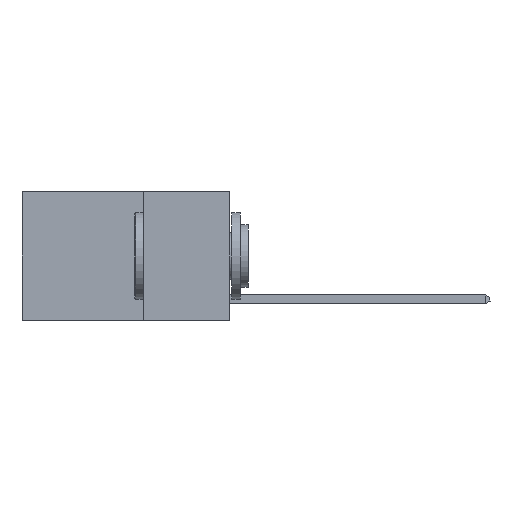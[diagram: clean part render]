
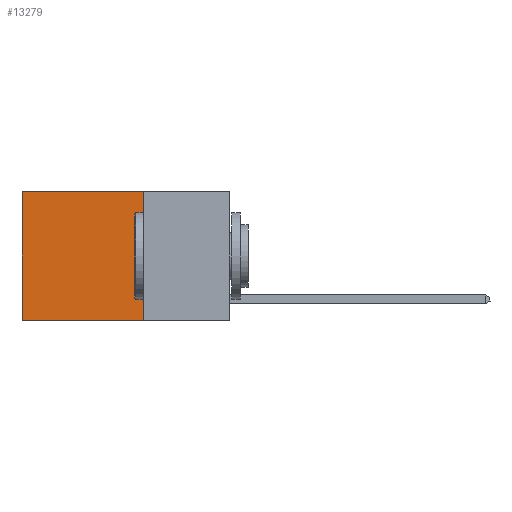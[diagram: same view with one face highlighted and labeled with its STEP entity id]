
A CAD part, left-side view. The second image highlights one B-rep face of the part: STEP entity #13279.
In plain terms, the highlighted planar face has unit normal (-1, 0, 0).
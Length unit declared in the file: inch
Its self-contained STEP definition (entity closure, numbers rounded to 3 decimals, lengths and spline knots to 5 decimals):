
#84 = VERTEX_POINT ( 'NONE', #3291 ) ;
#549 = LINE ( 'NONE', #4845, #22492 ) ;
#678 = CARTESIAN_POINT ( 'NONE',  ( 0.2625, 0.25, -0.37 ) ) ;
#924 = DIRECTION ( 'NONE',  ( 0., 1., 0. ) ) ;
#1273 = VERTEX_POINT ( 'NONE', #23144 ) ;
#1702 = ORIENTED_EDGE ( 'NONE', *, *, #26245, .F. ) ;
#2049 = CARTESIAN_POINT ( 'NONE',  ( 0.2625, 0.25, 0. ) ) ;
#2147 = AXIS2_PLACEMENT_3D ( 'NONE', #2049, #10299, #3941 ) ;
#2783 = EDGE_CURVE ( 'NONE', #18845, #5482, #21768, .T. ) ;
#3242 = CARTESIAN_POINT ( 'NONE',  ( 0.2625, 0.25, 0. ) ) ;
#3291 = CARTESIAN_POINT ( 'NONE',  ( 0.2625, 0.6, -0.37 ) ) ;
#3941 = DIRECTION ( 'NONE',  ( 0., 0., -1. ) ) ;
#4845 = CARTESIAN_POINT ( 'NONE',  ( 0.2625, 0.25, -0.37 ) ) ;
#5482 = VERTEX_POINT ( 'NONE', #678 ) ;
#6675 = EDGE_CURVE ( 'NONE', #1273, #84, #17827, .T. ) ;
#8656 = VECTOR ( 'NONE', #19733, 39.37008 ) ;
#8778 = DIRECTION ( 'NONE',  ( 0., 1., 0. ) ) ;
#9307 = ORIENTED_EDGE ( 'NONE', *, *, #20767, .T. ) ;
#10006 = CARTESIAN_POINT ( 'NONE',  ( 0.2625, 0.6, 0. ) ) ;
#10299 = DIRECTION ( 'NONE',  ( 1., 0., 0. ) ) ;
#13279 = ADVANCED_FACE ( 'NONE', ( #22460 ), #20853, .F. ) ;
#13759 = DIRECTION ( 'NONE',  ( 0., 0., -1. ) ) ;
#15362 = CARTESIAN_POINT ( 'NONE',  ( 0.2625, 0.25, 0. ) ) ;
#15651 = EDGE_LOOP ( 'NONE', ( #25952, #1702, #21715, #9307 ) ) ;
#17827 = LINE ( 'NONE', #10006, #20388 ) ;
#18845 = VERTEX_POINT ( 'NONE', #23795 ) ;
#19733 = DIRECTION ( 'NONE',  ( 0., 0., -1. ) ) ;
#20388 = VECTOR ( 'NONE', #13759, 39.37008 ) ;
#20767 = EDGE_CURVE ( 'NONE', #18845, #1273, #21066, .T. ) ;
#20853 = PLANE ( 'NONE',  #2147 ) ;
#21066 = LINE ( 'NONE', #15362, #26256 ) ;
#21715 = ORIENTED_EDGE ( 'NONE', *, *, #2783, .F. ) ;
#21768 = LINE ( 'NONE', #3242, #8656 ) ;
#22460 = FACE_OUTER_BOUND ( 'NONE', #15651, .T. ) ;
#22492 = VECTOR ( 'NONE', #8778, 39.37008 ) ;
#23144 = CARTESIAN_POINT ( 'NONE',  ( 0.2625, 0.6, 0. ) ) ;
#23795 = CARTESIAN_POINT ( 'NONE',  ( 0.2625, 0.25, 0. ) ) ;
#25952 = ORIENTED_EDGE ( 'NONE', *, *, #6675, .T. ) ;
#26245 = EDGE_CURVE ( 'NONE', #5482, #84, #549, .T. ) ;
#26256 = VECTOR ( 'NONE', #924, 39.37008 ) ;
